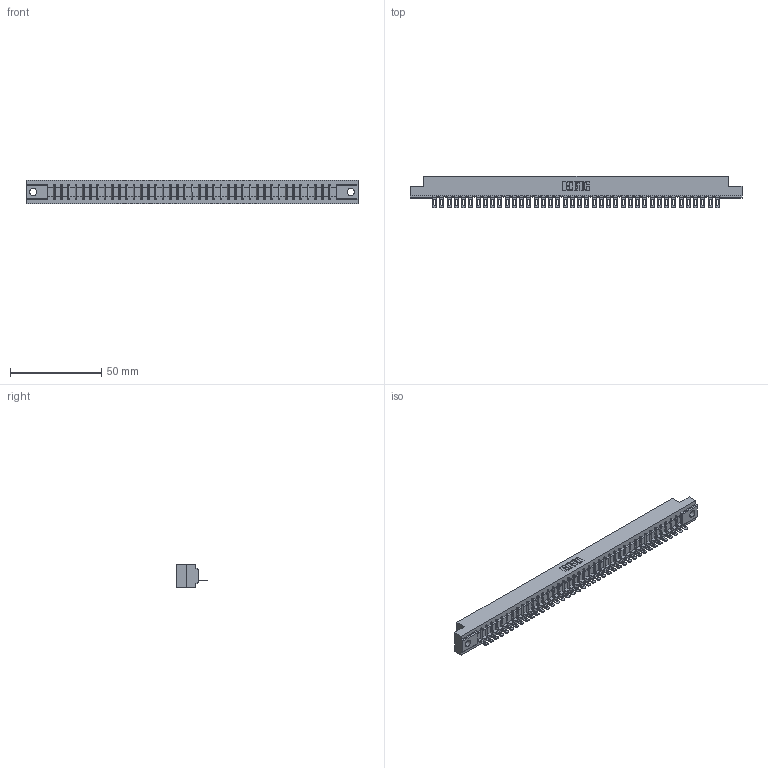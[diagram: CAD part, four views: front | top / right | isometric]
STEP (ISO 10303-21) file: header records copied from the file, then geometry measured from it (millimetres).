
FILE_DESCRIPTION (( 'STEP AP203' ), '1' );
FILE_NAME ('307-040-501-104.STEP', '2019-09-05T10:11:40', ( '' ), ( '' ), 'SwSTEP 2.0', 'SolidWorks 2016', '' );
FILE_SCHEMA (( 'CONFIG_CONTROL_DESIGN' ));
Length unit declared in the file: inch
Products named in the file (3): 307 Part_.156 Dia Mounting Holes; 307-290-002_501; 307-040-501-104
Assembly tree (41 placements, depth 2):
  307-040-501-104
    307 Part_.156 Dia Mounting Holes
    307-290-002_501  x40
Bounding box: 181.51 x 17.42 x 12.7 mm (x, y, z)
Volume: 19337.7 mm3; surface area: 24376.5 mm2
Topology: 41 solids, 41 shells, 3213 faces, 9879 edges, 6474 vertices
Faces by surface type: plane 1844, cylinder 1287, sphere 82
Entity records: 35750 total; most frequent: CARTESIAN_POINT 6034, ORIENTED_EDGE 6022, DIRECTION 5859, EDGE_CURVE 3011, VECTOR 2309, LINE 2309, VERTEX_POINT 1950, AXIS2_PLACEMENT_3D 1775
